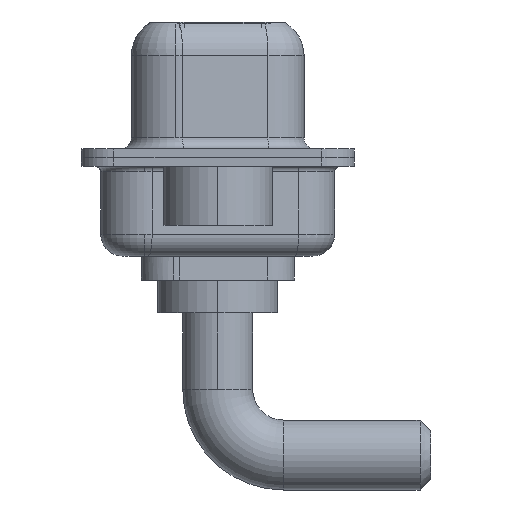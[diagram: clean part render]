
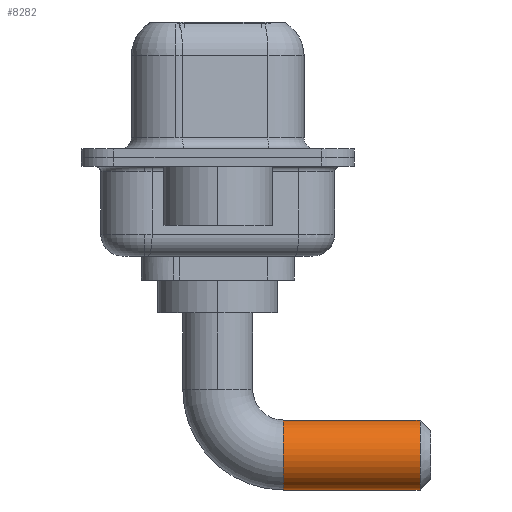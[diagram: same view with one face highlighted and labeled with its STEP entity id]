
A CAD part, left-side view. The second image highlights one B-rep face of the part: STEP entity #8282.
In plain terms, the highlighted cylindrical face has radius 1.6 mm (diameter 3.2 mm), a partial arc.
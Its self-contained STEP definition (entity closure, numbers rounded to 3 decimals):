
#460 = VERTEX_POINT ( 'NONE', #12474 ) ;
#504 = AXIS2_PLACEMENT_3D ( 'NONE', #12843, #5709, #3613 ) ;
#663 = ORIENTED_EDGE ( 'NONE', *, *, #2406, .T. ) ;
#818 = ORIENTED_EDGE ( 'NONE', *, *, #5852, .T. ) ;
#1644 = CYLINDRICAL_SURFACE ( 'NONE', #504, 1.6 ) ;
#2406 = EDGE_CURVE ( 'NONE', #460, #6869, #10906, .T. ) ;
#3293 = LINE ( 'NONE', #10322, #7646 ) ;
#3471 = CIRCLE ( 'NONE', #11221, 1.6 ) ;
#3613 = DIRECTION ( 'NONE',  ( 0., 0., -1. ) ) ;
#3760 = ORIENTED_EDGE ( 'NONE', *, *, #10096, .F. ) ;
#4986 = CARTESIAN_POINT ( 'NONE',  ( 0., -3., -6.5 ) ) ;
#5406 = LINE ( 'NONE', #11748, #12264 ) ;
#5709 = DIRECTION ( 'NONE',  ( 0., -1., 0. ) ) ;
#5852 = EDGE_CURVE ( 'NONE', #6853, #9239, #3471, .T. ) ;
#6807 = DIRECTION ( 'NONE',  ( -1., 0., 0. ) ) ;
#6853 = VERTEX_POINT ( 'NONE', #12434 ) ;
#6869 = VERTEX_POINT ( 'NONE', #11418 ) ;
#7074 = DIRECTION ( 'NONE',  ( 0., -1., 0. ) ) ;
#7281 = DIRECTION ( 'NONE',  ( 0., 0., -1. ) ) ;
#7531 = EDGE_LOOP ( 'NONE', ( #3760, #818, #8204, #663 ) ) ;
#7646 = VECTOR ( 'NONE', #8154, 1000. ) ;
#8154 = DIRECTION ( 'NONE',  ( 0., -1., 0. ) ) ;
#8204 = ORIENTED_EDGE ( 'NONE', *, *, #9427, .T. ) ;
#8282 = ADVANCED_FACE ( 'NONE', ( #9628 ), #1644, .T. ) ;
#9239 = VERTEX_POINT ( 'NONE', #12876 ) ;
#9427 = EDGE_CURVE ( 'NONE', #9239, #460, #3293, .T. ) ;
#9606 = DIRECTION ( 'NONE',  ( 0., -1., 0. ) ) ;
#9628 = FACE_OUTER_BOUND ( 'NONE', #7531, .T. ) ;
#10096 = EDGE_CURVE ( 'NONE', #6853, #6869, #5406, .T. ) ;
#10322 = CARTESIAN_POINT ( 'NONE',  ( 0., -3., -8.1 ) ) ;
#10450 = DIRECTION ( 'NONE',  ( 0., 1., 0. ) ) ;
#10906 = CIRCLE ( 'NONE', #11332, 1.6 ) ;
#11221 = AXIS2_PLACEMENT_3D ( 'NONE', #4986, #7074, #6807 ) ;
#11332 = AXIS2_PLACEMENT_3D ( 'NONE', #12135, #10450, #7281 ) ;
#11418 = CARTESIAN_POINT ( 'NONE',  ( 0., -9.25, -4.9 ) ) ;
#11748 = CARTESIAN_POINT ( 'NONE',  ( 0., -3., -4.9 ) ) ;
#12135 = CARTESIAN_POINT ( 'NONE',  ( 0., -9.25, -6.5 ) ) ;
#12264 = VECTOR ( 'NONE', #9606, 1000. ) ;
#12434 = CARTESIAN_POINT ( 'NONE',  ( 0., -3., -4.9 ) ) ;
#12474 = CARTESIAN_POINT ( 'NONE',  ( 0., -9.25, -8.1 ) ) ;
#12843 = CARTESIAN_POINT ( 'NONE',  ( 0., -3., -6.5 ) ) ;
#12876 = CARTESIAN_POINT ( 'NONE',  ( 0., -3., -8.1 ) ) ;
